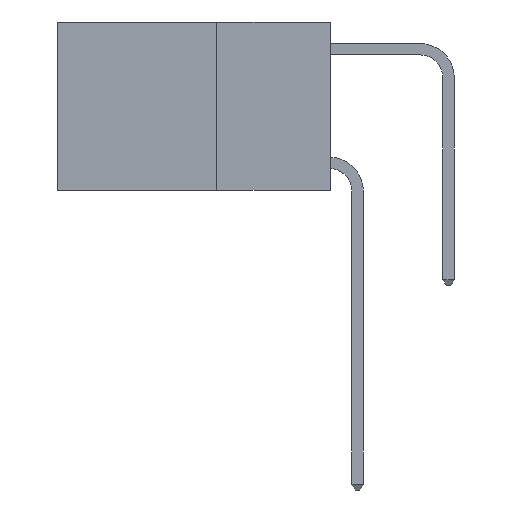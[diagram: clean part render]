
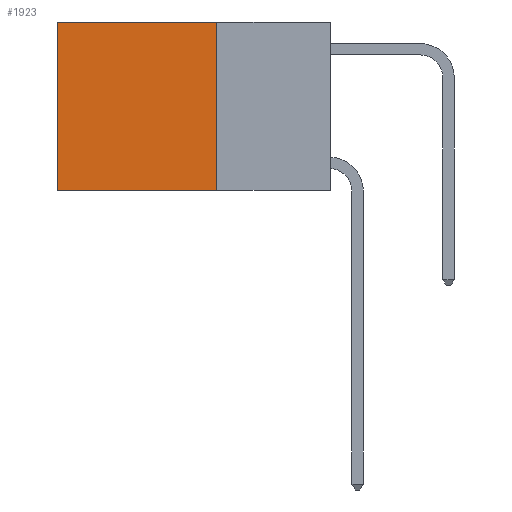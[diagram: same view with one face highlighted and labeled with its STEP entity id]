
A CAD part, left-side view. The second image highlights one B-rep face of the part: STEP entity #1923.
In plain terms, the highlighted planar face has unit normal (-1, 0, 0).
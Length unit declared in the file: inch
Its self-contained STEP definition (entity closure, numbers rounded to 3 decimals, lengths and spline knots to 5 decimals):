
#588 = VERTEX_POINT ( 'NONE', #6874 ) ;
#601 = VERTEX_POINT ( 'NONE', #2263 ) ;
#801 = FACE_OUTER_BOUND ( 'NONE', #9333, .T. ) ;
#861 = DIRECTION ( 'NONE',  ( 0., 1., 0. ) ) ;
#1093 = ORIENTED_EDGE ( 'NONE', *, *, #10343, .T. ) ;
#1325 = VERTEX_POINT ( 'NONE', #7183 ) ;
#1816 = DIRECTION ( 'NONE',  ( 0., 0., -1. ) ) ;
#1923 = ADVANCED_FACE ( 'NONE', ( #801 ), #9188, .F. ) ;
#2156 = EDGE_CURVE ( 'NONE', #1325, #601, #3594, .T. ) ;
#2263 = CARTESIAN_POINT ( 'NONE',  ( 0.2625, 0.6, -0.37 ) ) ;
#3594 = LINE ( 'NONE', #7911, #8316 ) ;
#3753 = ORIENTED_EDGE ( 'NONE', *, *, #4389, .F. ) ;
#3894 = ORIENTED_EDGE ( 'NONE', *, *, #6230, .F. ) ;
#3967 = CARTESIAN_POINT ( 'NONE',  ( 0.2625, 0.25, 0. ) ) ;
#4164 = AXIS2_PLACEMENT_3D ( 'NONE', #9373, #9164, #9151 ) ;
#4389 = EDGE_CURVE ( 'NONE', #588, #10113, #7529, .T. ) ;
#4727 = VECTOR ( 'NONE', #1816, 39.37008 ) ;
#5041 = LINE ( 'NONE', #3967, #5320 ) ;
#5320 = VECTOR ( 'NONE', #5853, 39.37008 ) ;
#5564 = CARTESIAN_POINT ( 'NONE',  ( 0.2625, 0.25, -0.37 ) ) ;
#5690 = CARTESIAN_POINT ( 'NONE',  ( 0.2625, 0.25, -0.37 ) ) ;
#5853 = DIRECTION ( 'NONE',  ( 0., 1., 0. ) ) ;
#6230 = EDGE_CURVE ( 'NONE', #10113, #601, #11298, .T. ) ;
#6874 = CARTESIAN_POINT ( 'NONE',  ( 0.2625, 0.25, 0. ) ) ;
#7183 = CARTESIAN_POINT ( 'NONE',  ( 0.2625, 0.6, 0. ) ) ;
#7529 = LINE ( 'NONE', #11346, #4727 ) ;
#7658 = DIRECTION ( 'NONE',  ( 0., 0., -1. ) ) ;
#7911 = CARTESIAN_POINT ( 'NONE',  ( 0.2625, 0.6, 0. ) ) ;
#8316 = VECTOR ( 'NONE', #7658, 39.37008 ) ;
#8799 = VECTOR ( 'NONE', #861, 39.37008 ) ;
#9151 = DIRECTION ( 'NONE',  ( 0., 0., -1. ) ) ;
#9164 = DIRECTION ( 'NONE',  ( 1., 0., 0. ) ) ;
#9188 = PLANE ( 'NONE',  #4164 ) ;
#9333 = EDGE_LOOP ( 'NONE', ( #10888, #3894, #3753, #1093 ) ) ;
#9373 = CARTESIAN_POINT ( 'NONE',  ( 0.2625, 0.25, 0. ) ) ;
#10113 = VERTEX_POINT ( 'NONE', #5564 ) ;
#10343 = EDGE_CURVE ( 'NONE', #588, #1325, #5041, .T. ) ;
#10888 = ORIENTED_EDGE ( 'NONE', *, *, #2156, .T. ) ;
#11298 = LINE ( 'NONE', #5690, #8799 ) ;
#11346 = CARTESIAN_POINT ( 'NONE',  ( 0.2625, 0.25, 0. ) ) ;
